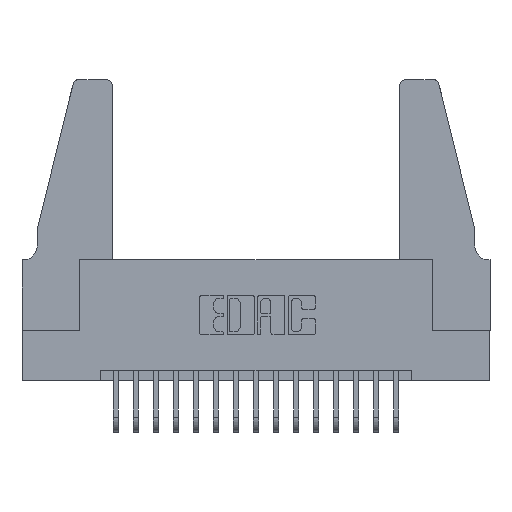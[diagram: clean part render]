
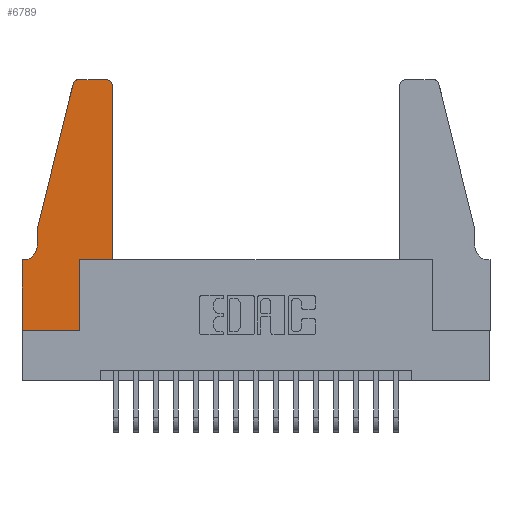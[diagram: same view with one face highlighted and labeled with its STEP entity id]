
A CAD part, top view. The second image highlights one B-rep face of the part: STEP entity #6789.
In plain terms, the highlighted planar face has unit normal (0, 0, 1).
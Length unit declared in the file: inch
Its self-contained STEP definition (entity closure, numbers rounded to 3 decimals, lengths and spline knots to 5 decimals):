
#504 = LINE ( 'NONE', #9324, #14251 ) ;
#846 = DIRECTION ( 'NONE',  ( 1., 0., 0. ) ) ;
#1093 = ORIENTED_EDGE ( 'NONE', *, *, #11578, .T. ) ;
#1242 = CARTESIAN_POINT ( 'NONE',  ( 0., 0., 0.37 ) ) ;
#1263 = VECTOR ( 'NONE', #7228, 39.37008 ) ;
#1342 = EDGE_CURVE ( 'NONE', #17004, #10753, #2899, .T. ) ;
#1577 = CARTESIAN_POINT ( 'NONE',  ( 0.2865, 0.35, 0.37 ) ) ;
#1708 = LINE ( 'NONE', #4538, #14978 ) ;
#2568 = VERTEX_POINT ( 'NONE', #15698 ) ;
#2633 = DIRECTION ( 'NONE',  ( 1., 0., 0. ) ) ;
#2697 = CARTESIAN_POINT ( 'NONE',  ( 0.2865, 0., 0.37 ) ) ;
#2899 = LINE ( 'NONE', #12989, #16493 ) ;
#3351 = VERTEX_POINT ( 'NONE', #3967 ) ;
#3583 = PLANE ( 'NONE',  #14417 ) ;
#3595 = VECTOR ( 'NONE', #6199, 39.37008 ) ;
#3967 = CARTESIAN_POINT ( 'NONE',  ( 0.0755, 0.5, 0.37 ) ) ;
#4024 = LINE ( 'NONE', #1242, #14098 ) ;
#4145 = ORIENTED_EDGE ( 'NONE', *, *, #5873, .T. ) ;
#4259 = VECTOR ( 'NONE', #15728, 39.37008 ) ;
#4310 = DIRECTION ( 'NONE',  ( 0., 0., -1. ) ) ;
#4468 = ORIENTED_EDGE ( 'NONE', *, *, #13095, .T. ) ;
#4470 = DIRECTION ( 'NONE',  ( -1., 0., 0. ) ) ;
#4495 = ORIENTED_EDGE ( 'NONE', *, *, #7027, .T. ) ;
#4538 = CARTESIAN_POINT ( 'NONE',  ( 0.0755, 0.5, 0.37 ) ) ;
#4731 = EDGE_CURVE ( 'NONE', #15694, #5856, #5307, .T. ) ;
#4768 = DIRECTION ( 'NONE',  ( 0., 0., 1. ) ) ;
#5307 = LINE ( 'NONE', #15149, #8432 ) ;
#5385 = VERTEX_POINT ( 'NONE', #12606 ) ;
#5589 = CARTESIAN_POINT ( 'NONE',  ( 0.4505, 0.35, 0.37 ) ) ;
#5657 = CARTESIAN_POINT ( 'NONE',  ( 0.4205, 1.25, 0.37 ) ) ;
#5721 = EDGE_CURVE ( 'NONE', #16830, #15062, #4024, .T. ) ;
#5762 = CARTESIAN_POINT ( 'NONE',  ( 0.2605, 1.25, 0.37 ) ) ;
#5856 = VERTEX_POINT ( 'NONE', #5589 ) ;
#5873 = EDGE_CURVE ( 'NONE', #2568, #17004, #8594, .T. ) ;
#5888 = VERTEX_POINT ( 'NONE', #5657 ) ;
#6199 = DIRECTION ( 'NONE',  ( 0., 1., 0. ) ) ;
#6203 = VERTEX_POINT ( 'NONE', #14066 ) ;
#6281 = DIRECTION ( 'NONE',  ( 1., 0., 0. ) ) ;
#6334 = ORIENTED_EDGE ( 'NONE', *, *, #1342, .T. ) ;
#6589 = CARTESIAN_POINT ( 'NONE',  ( 0.4505, 0.35, 0.37 ) ) ;
#6789 = ADVANCED_FACE ( 'NONE', ( #10994 ), #3583, .T. ) ;
#7027 = EDGE_CURVE ( 'NONE', #14194, #3351, #504, .T. ) ;
#7228 = DIRECTION ( 'NONE',  ( 0., -1., 0. ) ) ;
#8432 = VECTOR ( 'NONE', #13820, 39.37008 ) ;
#8447 = LINE ( 'NONE', #13731, #1263 ) ;
#8594 = CIRCLE ( 'NONE', #12756, 0.07 ) ;
#8758 = ORIENTED_EDGE ( 'NONE', *, *, #4731, .T. ) ;
#8871 = CARTESIAN_POINT ( 'NONE',  ( 0., 0.35, 0.37 ) ) ;
#8912 = DIRECTION ( 'NONE',  ( 0., 0., 1. ) ) ;
#9189 = EDGE_CURVE ( 'NONE', #5385, #14194, #14987, .T. ) ;
#9324 = CARTESIAN_POINT ( 'NONE',  ( 0.0755, 0.5, 0.37 ) ) ;
#10080 = CARTESIAN_POINT ( 'NONE',  ( 0.0055, 0.35, 0.37 ) ) ;
#10286 = EDGE_CURVE ( 'NONE', #3351, #2568, #1708, .T. ) ;
#10295 = EDGE_CURVE ( 'NONE', #10753, #16830, #8447, .T. ) ;
#10322 = ORIENTED_EDGE ( 'NONE', *, *, #9189, .T. ) ;
#10441 = DIRECTION ( 'NONE',  ( -1., 0., 0. ) ) ;
#10753 = VERTEX_POINT ( 'NONE', #14828 ) ;
#10789 = VECTOR ( 'NONE', #4470, 39.37008 ) ;
#10994 = FACE_OUTER_BOUND ( 'NONE', #11375, .T. ) ;
#11142 = ORIENTED_EDGE ( 'NONE', *, *, #10295, .T. ) ;
#11375 = EDGE_LOOP ( 'NONE', ( #15523, #10322, #4495, #12921, #4145, #6334, #11142, #13875, #1093, #8758, #4468, #16442 ) ) ;
#11578 = EDGE_CURVE ( 'NONE', #15062, #15694, #14097, .T. ) ;
#12186 = CARTESIAN_POINT ( 'NONE',  ( 0.0055, 0.42, 0.37 ) ) ;
#12200 = EDGE_CURVE ( 'NONE', #6203, #5888, #14290, .T. ) ;
#12290 = CARTESIAN_POINT ( 'NONE',  ( 0., 0., 0.37 ) ) ;
#12606 = CARTESIAN_POINT ( 'NONE',  ( 0.284, 1.25, 0.37 ) ) ;
#12651 = CARTESIAN_POINT ( 'NONE',  ( 0.4205, 1.22, 0.37 ) ) ;
#12756 = AXIS2_PLACEMENT_3D ( 'NONE', #12186, #4310, #13499 ) ;
#12921 = ORIENTED_EDGE ( 'NONE', *, *, #10286, .T. ) ;
#12989 = CARTESIAN_POINT ( 'NONE',  ( 0.0755, 0.35, 0.37 ) ) ;
#13095 = EDGE_CURVE ( 'NONE', #5856, #6203, #14346, .T. ) ;
#13499 = DIRECTION ( 'NONE',  ( -1., 0., 0. ) ) ;
#13731 = CARTESIAN_POINT ( 'NONE',  ( 0., 0., 0.37 ) ) ;
#13798 = AXIS2_PLACEMENT_3D ( 'NONE', #12651, #4768, #13956 ) ;
#13820 = DIRECTION ( 'NONE',  ( 1., 0., 0. ) ) ;
#13875 = ORIENTED_EDGE ( 'NONE', *, *, #5721, .T. ) ;
#13956 = DIRECTION ( 'NONE',  ( 1., 0., 0. ) ) ;
#13978 = CARTESIAN_POINT ( 'NONE',  ( 0.2865, 0.35, 0.37 ) ) ;
#14066 = CARTESIAN_POINT ( 'NONE',  ( 0.4505, 1.22, 0.37 ) ) ;
#14097 = LINE ( 'NONE', #13978, #3595 ) ;
#14098 = VECTOR ( 'NONE', #2633, 39.37008 ) ;
#14115 = DIRECTION ( 'NONE',  ( 0., 0., 1. ) ) ;
#14194 = VERTEX_POINT ( 'NONE', #15423 ) ;
#14251 = VECTOR ( 'NONE', #15869, 39.37008 ) ;
#14259 = LINE ( 'NONE', #5762, #10789 ) ;
#14290 = CIRCLE ( 'NONE', #13798, 0.03 ) ;
#14346 = LINE ( 'NONE', #6589, #4259 ) ;
#14417 = AXIS2_PLACEMENT_3D ( 'NONE', #8871, #14115, #6281 ) ;
#14440 = AXIS2_PLACEMENT_3D ( 'NONE', #16704, #8912, #846 ) ;
#14828 = CARTESIAN_POINT ( 'NONE',  ( 0., 0.35, 0.37 ) ) ;
#14978 = VECTOR ( 'NONE', #15054, 39.37008 ) ;
#14987 = CIRCLE ( 'NONE', #14440, 0.03 ) ;
#15054 = DIRECTION ( 'NONE',  ( 0., -1., 0. ) ) ;
#15062 = VERTEX_POINT ( 'NONE', #2697 ) ;
#15149 = CARTESIAN_POINT ( 'NONE',  ( 0.4505, 0.35, 0.37 ) ) ;
#15257 = EDGE_CURVE ( 'NONE', #5888, #5385, #14259, .T. ) ;
#15423 = CARTESIAN_POINT ( 'NONE',  ( 0.25487, 1.22718, 0.37 ) ) ;
#15523 = ORIENTED_EDGE ( 'NONE', *, *, #15257, .T. ) ;
#15694 = VERTEX_POINT ( 'NONE', #1577 ) ;
#15698 = CARTESIAN_POINT ( 'NONE',  ( 0.0755, 0.42, 0.37 ) ) ;
#15728 = DIRECTION ( 'NONE',  ( 0., 1., 0. ) ) ;
#15869 = DIRECTION ( 'NONE',  ( -0.239, -0.971, 0. ) ) ;
#16442 = ORIENTED_EDGE ( 'NONE', *, *, #12200, .T. ) ;
#16493 = VECTOR ( 'NONE', #10441, 39.37008 ) ;
#16704 = CARTESIAN_POINT ( 'NONE',  ( 0.284, 1.22, 0.37 ) ) ;
#16830 = VERTEX_POINT ( 'NONE', #12290 ) ;
#17004 = VERTEX_POINT ( 'NONE', #10080 ) ;
